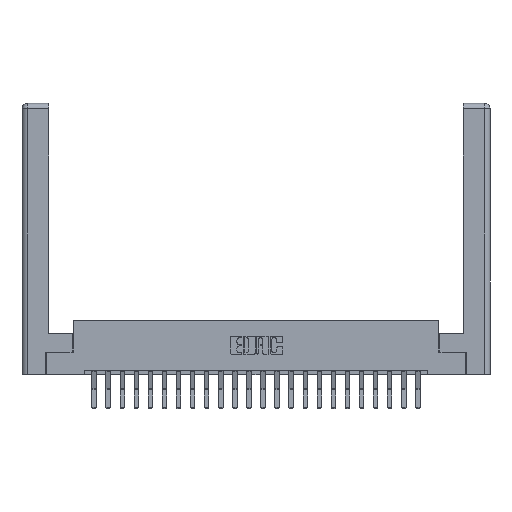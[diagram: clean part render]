
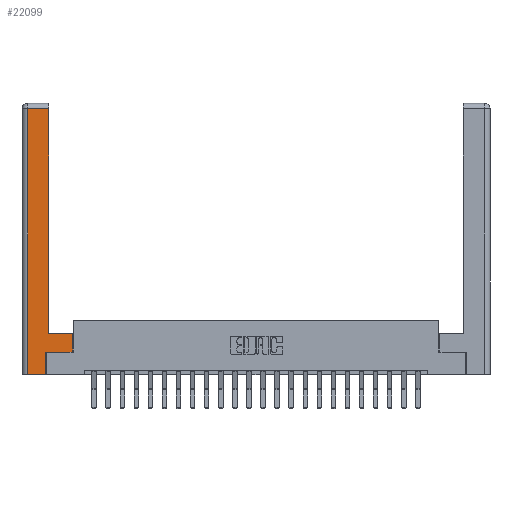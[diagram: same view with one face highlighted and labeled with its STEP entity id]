
A CAD part, top view. The second image highlights one B-rep face of the part: STEP entity #22099.
In plain terms, the highlighted planar face has unit normal (0, 0, 1).
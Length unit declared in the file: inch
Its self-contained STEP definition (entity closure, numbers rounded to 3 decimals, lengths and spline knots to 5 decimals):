
#229 = DIRECTION ( 'NONE',  ( 0., 1., 0. ) ) ;
#845 = AXIS2_PLACEMENT_3D ( 'NONE', #5852, #13406, #22405 ) ;
#868 = CARTESIAN_POINT ( 'NONE',  ( 0.0615, 0., 0. ) ) ;
#1549 = EDGE_CURVE ( 'NONE', #8177, #20960, #19275, .T. ) ;
#2258 = EDGE_CURVE ( 'NONE', #14077, #3213, #5553, .T. ) ;
#2393 = CARTESIAN_POINT ( 'NONE',  ( 0.0615, 2.94, 0. ) ) ;
#2752 = CARTESIAN_POINT ( 'NONE',  ( 0.565, 0.245, 0. ) ) ;
#3119 = VECTOR ( 'NONE', #11026, 39.37008 ) ;
#3213 = VERTEX_POINT ( 'NONE', #20588 ) ;
#3289 = CARTESIAN_POINT ( 'NONE',  ( 0.565, 0.45, 0. ) ) ;
#3683 = VECTOR ( 'NONE', #7863, 39.37008 ) ;
#4334 = EDGE_CURVE ( 'NONE', #21683, #8177, #7946, .T. ) ;
#4473 = VERTEX_POINT ( 'NONE', #20643 ) ;
#4573 = EDGE_CURVE ( 'NONE', #20960, #14077, #21112, .T. ) ;
#4786 = VECTOR ( 'NONE', #21537, 39.37008 ) ;
#5553 = LINE ( 'NONE', #6911, #16684 ) ;
#5852 = CARTESIAN_POINT ( 'NONE',  ( 0., 0., 0. ) ) ;
#6911 = CARTESIAN_POINT ( 'NONE',  ( 0.265, 0.245, 0. ) ) ;
#7863 = DIRECTION ( 'NONE',  ( -1., 0., 0. ) ) ;
#7946 = LINE ( 'NONE', #20253, #3119 ) ;
#8099 = EDGE_CURVE ( 'NONE', #21536, #21683, #15175, .T. ) ;
#8177 = VERTEX_POINT ( 'NONE', #2393 ) ;
#8697 = CARTESIAN_POINT ( 'NONE',  ( 0.265, 0., 0. ) ) ;
#8918 = CARTESIAN_POINT ( 'NONE',  ( 0.565, 0.245, 0. ) ) ;
#9700 = EDGE_CURVE ( 'NONE', #4473, #21536, #18188, .T. ) ;
#10273 = DIRECTION ( 'NONE',  ( 0., -1., 0. ) ) ;
#10336 = EDGE_CURVE ( 'NONE', #3213, #15435, #23379, .T. ) ;
#10557 = ORIENTED_EDGE ( 'NONE', *, *, #1549, .T. ) ;
#11026 = DIRECTION ( 'NONE',  ( -1., 0., 0. ) ) ;
#11218 = ORIENTED_EDGE ( 'NONE', *, *, #14127, .T. ) ;
#11653 = DIRECTION ( 'NONE',  ( 1., 0., 0. ) ) ;
#12233 = ORIENTED_EDGE ( 'NONE', *, *, #2258, .T. ) ;
#12353 = ORIENTED_EDGE ( 'NONE', *, *, #8099, .T. ) ;
#13406 = DIRECTION ( 'NONE',  ( 0., 0., -1. ) ) ;
#13792 = EDGE_LOOP ( 'NONE', ( #12353, #19081, #10557, #18680, #12233, #20351, #11218, #15491 ) ) ;
#14077 = VERTEX_POINT ( 'NONE', #8697 ) ;
#14127 = EDGE_CURVE ( 'NONE', #15435, #4473, #19161, .T. ) ;
#15092 = CARTESIAN_POINT ( 'NONE',  ( 0.295, 0.45, 0. ) ) ;
#15153 = VECTOR ( 'NONE', #21322, 39.37008 ) ;
#15175 = LINE ( 'NONE', #16576, #16339 ) ;
#15435 = VERTEX_POINT ( 'NONE', #8918 ) ;
#15491 = ORIENTED_EDGE ( 'NONE', *, *, #9700, .T. ) ;
#15513 = CARTESIAN_POINT ( 'NONE',  ( 0.295, 0.45, 0. ) ) ;
#15712 = CARTESIAN_POINT ( 'NONE',  ( 0.295, 2.94, 0. ) ) ;
#15912 = VECTOR ( 'NONE', #11653, 39.37008 ) ;
#16339 = VECTOR ( 'NONE', #229, 39.37008 ) ;
#16576 = CARTESIAN_POINT ( 'NONE',  ( 0.295, 3., 0. ) ) ;
#16684 = VECTOR ( 'NONE', #17951, 39.37008 ) ;
#16727 = VECTOR ( 'NONE', #10273, 39.37008 ) ;
#17951 = DIRECTION ( 'NONE',  ( 0., 1., 0. ) ) ;
#18188 = LINE ( 'NONE', #15092, #3683 ) ;
#18680 = ORIENTED_EDGE ( 'NONE', *, *, #4573, .T. ) ;
#19081 = ORIENTED_EDGE ( 'NONE', *, *, #4334, .T. ) ;
#19161 = LINE ( 'NONE', #3289, #15153 ) ;
#19275 = LINE ( 'NONE', #868, #16727 ) ;
#19669 = CARTESIAN_POINT ( 'NONE',  ( 0.265, 0., 0. ) ) ;
#20253 = CARTESIAN_POINT ( 'NONE',  ( 0.0615, 2.94, 0. ) ) ;
#20351 = ORIENTED_EDGE ( 'NONE', *, *, #10336, .T. ) ;
#20588 = CARTESIAN_POINT ( 'NONE',  ( 0.265, 0.245, 0. ) ) ;
#20643 = CARTESIAN_POINT ( 'NONE',  ( 0.565, 0.45, 0. ) ) ;
#20960 = VERTEX_POINT ( 'NONE', #22683 ) ;
#21112 = LINE ( 'NONE', #19669, #4786 ) ;
#21322 = DIRECTION ( 'NONE',  ( 0., 1., 0. ) ) ;
#21536 = VERTEX_POINT ( 'NONE', #15513 ) ;
#21537 = DIRECTION ( 'NONE',  ( 1., 0., 0. ) ) ;
#21683 = VERTEX_POINT ( 'NONE', #15712 ) ;
#22099 = ADVANCED_FACE ( 'NONE', ( #22530 ), #22565, .F. ) ;
#22405 = DIRECTION ( 'NONE',  ( -1., 0., 0. ) ) ;
#22530 = FACE_OUTER_BOUND ( 'NONE', #13792, .T. ) ;
#22565 = PLANE ( 'NONE',  #845 ) ;
#22683 = CARTESIAN_POINT ( 'NONE',  ( 0.0615, 0., 0. ) ) ;
#23379 = LINE ( 'NONE', #2752, #15912 ) ;
